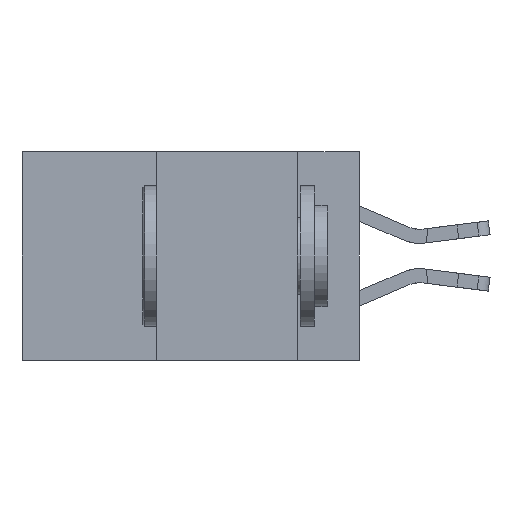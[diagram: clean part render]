
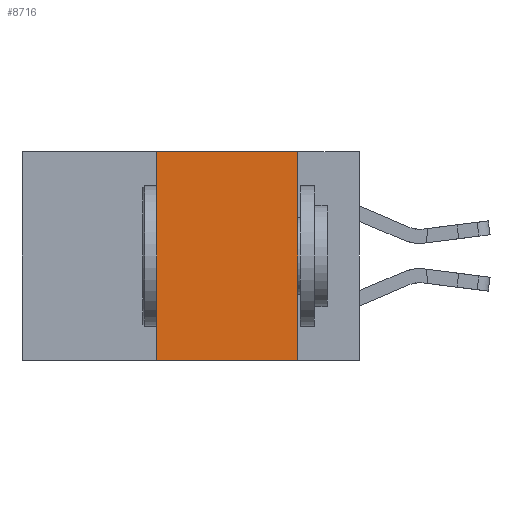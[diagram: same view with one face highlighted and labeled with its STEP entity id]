
A CAD part, left-side view. The second image highlights one B-rep face of the part: STEP entity #8716.
In plain terms, the highlighted planar face has unit normal (-1, 0, 0).
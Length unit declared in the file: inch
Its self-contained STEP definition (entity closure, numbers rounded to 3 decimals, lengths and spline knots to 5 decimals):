
#122 = EDGE_CURVE ( 'NONE', #5930, #7637, #13389, .T. ) ;
#153 = FACE_OUTER_BOUND ( 'NONE', #3104, .T. ) ;
#172 = CARTESIAN_POINT ( 'NONE',  ( 0., 0.36, 0. ) ) ;
#243 = DIRECTION ( 'NONE',  ( 0., -1., 0. ) ) ;
#1080 = VECTOR ( 'NONE', #6636, 39.37008 ) ;
#1543 = CARTESIAN_POINT ( 'NONE',  ( 0., 0.11, -0.37 ) ) ;
#1769 = DIRECTION ( 'NONE',  ( 0., -1., 0. ) ) ;
#2533 = ORIENTED_EDGE ( 'NONE', *, *, #5813, .F. ) ;
#2778 = CARTESIAN_POINT ( 'NONE',  ( 0., 0.6, 0. ) ) ;
#3104 = EDGE_LOOP ( 'NONE', ( #2533, #7769, #16705, #6438 ) ) ;
#3539 = CARTESIAN_POINT ( 'NONE',  ( 0., 0.36, 0. ) ) ;
#4413 = EDGE_CURVE ( 'NONE', #7637, #4708, #14447, .T. ) ;
#4708 = VERTEX_POINT ( 'NONE', #5144 ) ;
#5144 = CARTESIAN_POINT ( 'NONE',  ( 0., 0.11, 0. ) ) ;
#5297 = VECTOR ( 'NONE', #6768, 39.37008 ) ;
#5813 = EDGE_CURVE ( 'NONE', #4708, #16608, #11261, .T. ) ;
#5930 = VERTEX_POINT ( 'NONE', #7154 ) ;
#6056 = VECTOR ( 'NONE', #243, 39.37008 ) ;
#6438 = ORIENTED_EDGE ( 'NONE', *, *, #11236, .T. ) ;
#6636 = DIRECTION ( 'NONE',  ( 0., 0., -1. ) ) ;
#6768 = DIRECTION ( 'NONE',  ( 0., 0., 1. ) ) ;
#6806 = DIRECTION ( 'NONE',  ( 0., 0., -1. ) ) ;
#7061 = LINE ( 'NONE', #8226, #6056 ) ;
#7154 = CARTESIAN_POINT ( 'NONE',  ( 0., 0.36, -0.37 ) ) ;
#7637 = VERTEX_POINT ( 'NONE', #3539 ) ;
#7769 = ORIENTED_EDGE ( 'NONE', *, *, #4413, .F. ) ;
#7800 = VECTOR ( 'NONE', #1769, 39.37008 ) ;
#8226 = CARTESIAN_POINT ( 'NONE',  ( 0., 0.6, -0.37 ) ) ;
#8716 = ADVANCED_FACE ( 'NONE', ( #153 ), #11983, .F. ) ;
#9676 = CARTESIAN_POINT ( 'NONE',  ( 0., 0.6, 0. ) ) ;
#9854 = CARTESIAN_POINT ( 'NONE',  ( 0., 0.11, 0. ) ) ;
#11236 = EDGE_CURVE ( 'NONE', #5930, #16608, #7061, .T. ) ;
#11261 = LINE ( 'NONE', #9854, #1080 ) ;
#11983 = PLANE ( 'NONE',  #15544 ) ;
#13389 = LINE ( 'NONE', #172, #5297 ) ;
#14447 = LINE ( 'NONE', #9676, #7800 ) ;
#15544 = AXIS2_PLACEMENT_3D ( 'NONE', #2778, #16043, #6806 ) ;
#16043 = DIRECTION ( 'NONE',  ( 1., 0., 0. ) ) ;
#16608 = VERTEX_POINT ( 'NONE', #1543 ) ;
#16705 = ORIENTED_EDGE ( 'NONE', *, *, #122, .F. ) ;
